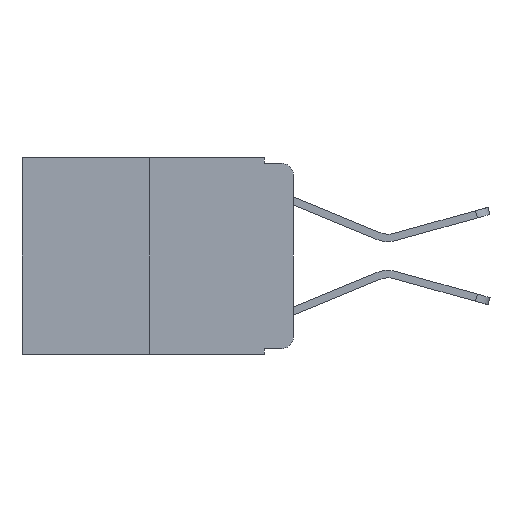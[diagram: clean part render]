
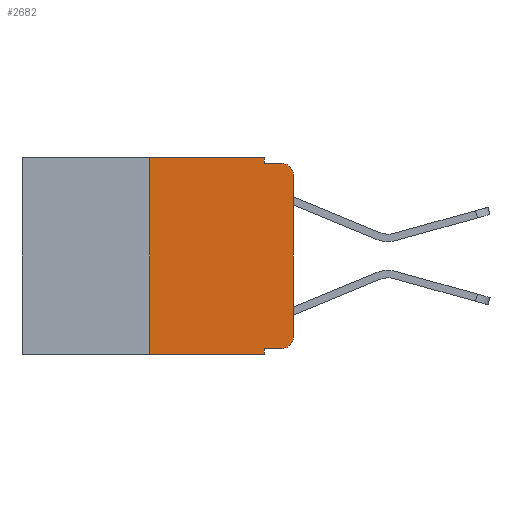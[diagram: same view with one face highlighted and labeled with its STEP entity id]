
A CAD part, left-side view. The second image highlights one B-rep face of the part: STEP entity #2682.
In plain terms, the highlighted planar face has unit normal (-1, 0, 0).
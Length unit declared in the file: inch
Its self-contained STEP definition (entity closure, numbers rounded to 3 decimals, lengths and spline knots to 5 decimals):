
#244 = CARTESIAN_POINT ( 'NONE',  ( 0., 0., -0.03 ) ) ;
#250 = ORIENTED_EDGE ( 'NONE', *, *, #744, .T. ) ;
#744 = EDGE_CURVE ( 'NONE', #10979, #7196, #11941, .T. ) ;
#918 = LINE ( 'NONE', #8197, #8473 ) ;
#1017 = LINE ( 'NONE', #14511, #3251 ) ;
#1104 = AXIS2_PLACEMENT_3D ( 'NONE', #16114, #1857, #4855 ) ;
#1341 = CARTESIAN_POINT ( 'NONE',  ( 0., 0.473, 0. ) ) ;
#1718 = CARTESIAN_POINT ( 'NONE',  ( 0., 0.051, -0.333 ) ) ;
#1857 = DIRECTION ( 'NONE',  ( -1., 0., 0. ) ) ;
#1963 = VERTEX_POINT ( 'NONE', #4291 ) ;
#2486 = CARTESIAN_POINT ( 'NONE',  ( 0., 0.25, 0. ) ) ;
#2572 = CARTESIAN_POINT ( 'NONE',  ( 0., 0.02, -0.01 ) ) ;
#2682 = ADVANCED_FACE ( 'NONE', ( #7409 ), #5787, .F. ) ;
#2875 = LINE ( 'NONE', #13783, #5770 ) ;
#3191 = VECTOR ( 'NONE', #16776, 39.37008 ) ;
#3251 = VECTOR ( 'NONE', #16046, 39.37008 ) ;
#3757 = CARTESIAN_POINT ( 'NONE',  ( 0., 0.02, -0.313 ) ) ;
#3796 = DIRECTION ( 'NONE',  ( 0., -1., 0. ) ) ;
#3931 = DIRECTION ( 'NONE',  ( 0., 0., -1. ) ) ;
#4228 = DIRECTION ( 'NONE',  ( 0., 0., -1. ) ) ;
#4291 = CARTESIAN_POINT ( 'NONE',  ( 0., 0., -0.313 ) ) ;
#4855 = DIRECTION ( 'NONE',  ( 0., 0., -1. ) ) ;
#4883 = CIRCLE ( 'NONE', #1104, 0.02 ) ;
#5036 = CARTESIAN_POINT ( 'NONE',  ( 0., 0.02, -0.333 ) ) ;
#5115 = EDGE_CURVE ( 'NONE', #7429, #5781, #4883, .T. ) ;
#5325 = EDGE_CURVE ( 'NONE', #7301, #9551, #8619, .T. ) ;
#5718 = LINE ( 'NONE', #14004, #12721 ) ;
#5770 = VECTOR ( 'NONE', #3796, 39.37008 ) ;
#5778 = AXIS2_PLACEMENT_3D ( 'NONE', #1341, #11218, #4228 ) ;
#5781 = VERTEX_POINT ( 'NONE', #2572 ) ;
#5787 = PLANE ( 'NONE',  #5778 ) ;
#6059 = VECTOR ( 'NONE', #13116, 39.37008 ) ;
#6435 = ORIENTED_EDGE ( 'NONE', *, *, #17722, .F. ) ;
#6454 = ORIENTED_EDGE ( 'NONE', *, *, #15102, .T. ) ;
#6590 = CARTESIAN_POINT ( 'NONE',  ( 0., 0.25, 0. ) ) ;
#6713 = DIRECTION ( 'NONE',  ( -1., 0., 0. ) ) ;
#6767 = ORIENTED_EDGE ( 'NONE', *, *, #14285, .F. ) ;
#6795 = DIRECTION ( 'NONE',  ( 0., 0., 1. ) ) ;
#6995 = EDGE_CURVE ( 'NONE', #10979, #7185, #1017, .T. ) ;
#7144 = DIRECTION ( 'NONE',  ( 0., 0., 1. ) ) ;
#7185 = VERTEX_POINT ( 'NONE', #11945 ) ;
#7196 = VERTEX_POINT ( 'NONE', #5036 ) ;
#7301 = VERTEX_POINT ( 'NONE', #14350 ) ;
#7409 = FACE_OUTER_BOUND ( 'NONE', #18071, .T. ) ;
#7429 = VERTEX_POINT ( 'NONE', #244 ) ;
#8197 = CARTESIAN_POINT ( 'NONE',  ( 0., 0.051, 0. ) ) ;
#8473 = VECTOR ( 'NONE', #3931, 39.37008 ) ;
#8476 = EDGE_CURVE ( 'NONE', #7196, #1963, #17011, .T. ) ;
#8600 = CARTESIAN_POINT ( 'NONE',  ( 0., 0.051, 0. ) ) ;
#8619 = LINE ( 'NONE', #2486, #17204 ) ;
#8973 = EDGE_CURVE ( 'NONE', #9551, #10172, #2875, .T. ) ;
#9357 = CARTESIAN_POINT ( 'NONE',  ( 0., 0.051, -0.333 ) ) ;
#9516 = ORIENTED_EDGE ( 'NONE', *, *, #8973, .F. ) ;
#9551 = VERTEX_POINT ( 'NONE', #6590 ) ;
#9656 = CARTESIAN_POINT ( 'NONE',  ( 0., 0.051, -0.01 ) ) ;
#9708 = CARTESIAN_POINT ( 'NONE',  ( 0., 0.051, -0.01 ) ) ;
#9735 = CARTESIAN_POINT ( 'NONE',  ( 0., 0.473, -0.343 ) ) ;
#10172 = VERTEX_POINT ( 'NONE', #8600 ) ;
#10660 = DIRECTION ( 'NONE',  ( 0., -1., 0. ) ) ;
#10979 = VERTEX_POINT ( 'NONE', #9357 ) ;
#11218 = DIRECTION ( 'NONE',  ( 1., 0., 0. ) ) ;
#11941 = LINE ( 'NONE', #1718, #6059 ) ;
#11945 = CARTESIAN_POINT ( 'NONE',  ( 0., 0.051, -0.343 ) ) ;
#12721 = VECTOR ( 'NONE', #7144, 39.37008 ) ;
#13116 = DIRECTION ( 'NONE',  ( 0., -1., 0. ) ) ;
#13226 = ORIENTED_EDGE ( 'NONE', *, *, #16487, .T. ) ;
#13407 = VERTEX_POINT ( 'NONE', #9708 ) ;
#13612 = DIRECTION ( 'NONE',  ( 0., 0., -1. ) ) ;
#13783 = CARTESIAN_POINT ( 'NONE',  ( 0., 0.473, 0. ) ) ;
#13867 = VECTOR ( 'NONE', #10660, 39.37008 ) ;
#14004 = CARTESIAN_POINT ( 'NONE',  ( 0., 0., 0. ) ) ;
#14285 = EDGE_CURVE ( 'NONE', #13407, #5781, #16071, .T. ) ;
#14350 = CARTESIAN_POINT ( 'NONE',  ( 0., 0.25, -0.343 ) ) ;
#14511 = CARTESIAN_POINT ( 'NONE',  ( 0., 0.051, 0. ) ) ;
#15014 = ORIENTED_EDGE ( 'NONE', *, *, #6995, .F. ) ;
#15102 = EDGE_CURVE ( 'NONE', #1963, #7429, #5718, .T. ) ;
#15468 = ORIENTED_EDGE ( 'NONE', *, *, #8476, .T. ) ;
#15772 = LINE ( 'NONE', #9735, #3191 ) ;
#16046 = DIRECTION ( 'NONE',  ( 0., 0., -1. ) ) ;
#16071 = LINE ( 'NONE', #9656, #13867 ) ;
#16114 = CARTESIAN_POINT ( 'NONE',  ( 0., 0.02, -0.03 ) ) ;
#16487 = EDGE_CURVE ( 'NONE', #7301, #7185, #15772, .T. ) ;
#16519 = ORIENTED_EDGE ( 'NONE', *, *, #5115, .T. ) ;
#16776 = DIRECTION ( 'NONE',  ( 0., -1., 0. ) ) ;
#17011 = CIRCLE ( 'NONE', #17347, 0.02 ) ;
#17204 = VECTOR ( 'NONE', #6795, 39.37008 ) ;
#17347 = AXIS2_PLACEMENT_3D ( 'NONE', #3757, #6713, #13612 ) ;
#17598 = ORIENTED_EDGE ( 'NONE', *, *, #5325, .F. ) ;
#17722 = EDGE_CURVE ( 'NONE', #10172, #13407, #918, .T. ) ;
#18071 = EDGE_LOOP ( 'NONE', ( #6454, #16519, #6767, #6435, #9516, #17598, #13226, #15014, #250, #15468 ) ) ;
